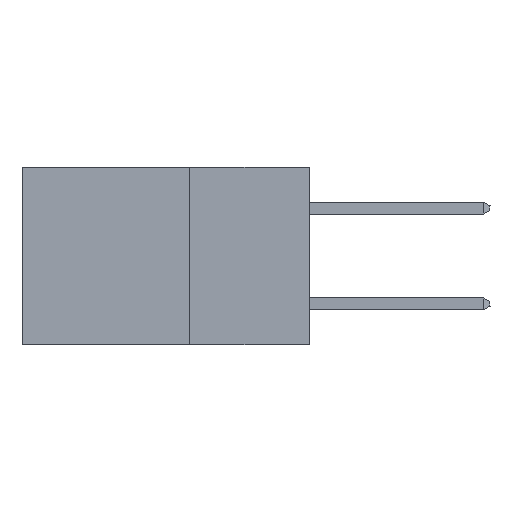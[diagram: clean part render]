
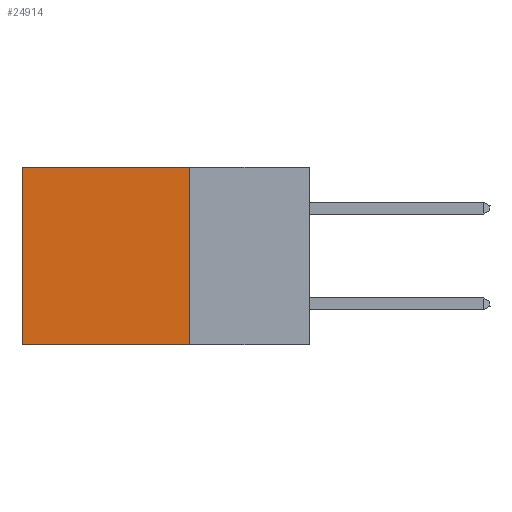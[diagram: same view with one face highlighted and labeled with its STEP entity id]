
A CAD part, left-side view. The second image highlights one B-rep face of the part: STEP entity #24914.
In plain terms, the highlighted planar face has unit normal (-1, 0, 0).
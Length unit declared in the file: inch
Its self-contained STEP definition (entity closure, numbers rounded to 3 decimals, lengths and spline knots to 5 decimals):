
#1022 = VECTOR ( 'NONE', #8077, 39.37008 ) ;
#1148 = EDGE_LOOP ( 'NONE', ( #30023, #14138, #10539, #38861 ) ) ;
#2577 = CARTESIAN_POINT ( 'NONE',  ( 0.2875, 0.25, 0. ) ) ;
#3048 = DIRECTION ( 'NONE',  ( 1., 0., 0. ) ) ;
#4821 = CARTESIAN_POINT ( 'NONE',  ( 0.2875, 0.6, -0.37 ) ) ;
#4990 = CARTESIAN_POINT ( 'NONE',  ( 0.2875, 0.6, 0. ) ) ;
#6301 = VERTEX_POINT ( 'NONE', #31669 ) ;
#6330 = EDGE_CURVE ( 'NONE', #6301, #18238, #8256, .T. ) ;
#6855 = VERTEX_POINT ( 'NONE', #31880 ) ;
#8077 = DIRECTION ( 'NONE',  ( 0., 0., -1. ) ) ;
#8256 = LINE ( 'NONE', #19258, #41388 ) ;
#8545 = DIRECTION ( 'NONE',  ( 0., 1., 0. ) ) ;
#9550 = EDGE_CURVE ( 'NONE', #39861, #6855, #35177, .T. ) ;
#10539 = ORIENTED_EDGE ( 'NONE', *, *, #35698, .F. ) ;
#11587 = CARTESIAN_POINT ( 'NONE',  ( 0.2875, 0.25, 0. ) ) ;
#14138 = ORIENTED_EDGE ( 'NONE', *, *, #6330, .F. ) ;
#17449 = VECTOR ( 'NONE', #8545, 39.37008 ) ;
#18238 = VERTEX_POINT ( 'NONE', #4821 ) ;
#19258 = CARTESIAN_POINT ( 'NONE',  ( 0.2875, 0.25, -0.37 ) ) ;
#19964 = AXIS2_PLACEMENT_3D ( 'NONE', #2577, #3048, #35775 ) ;
#24914 = ADVANCED_FACE ( 'NONE', ( #38401 ), #39150, .F. ) ;
#26422 = CARTESIAN_POINT ( 'NONE',  ( 0.2875, 0.25, 0. ) ) ;
#26456 = EDGE_CURVE ( 'NONE', #6855, #18238, #30261, .T. ) ;
#30023 = ORIENTED_EDGE ( 'NONE', *, *, #26456, .T. ) ;
#30261 = LINE ( 'NONE', #4990, #46245 ) ;
#30712 = LINE ( 'NONE', #26422, #1022 ) ;
#31669 = CARTESIAN_POINT ( 'NONE',  ( 0.2875, 0.25, -0.37 ) ) ;
#31880 = CARTESIAN_POINT ( 'NONE',  ( 0.2875, 0.6, 0. ) ) ;
#34214 = DIRECTION ( 'NONE',  ( 0., 0., -1. ) ) ;
#35177 = LINE ( 'NONE', #11587, #17449 ) ;
#35698 = EDGE_CURVE ( 'NONE', #39861, #6301, #30712, .T. ) ;
#35775 = DIRECTION ( 'NONE',  ( 0., 0., -1. ) ) ;
#37286 = CARTESIAN_POINT ( 'NONE',  ( 0.2875, 0.25, 0. ) ) ;
#38401 = FACE_OUTER_BOUND ( 'NONE', #1148, .T. ) ;
#38861 = ORIENTED_EDGE ( 'NONE', *, *, #9550, .T. ) ;
#39150 = PLANE ( 'NONE',  #19964 ) ;
#39861 = VERTEX_POINT ( 'NONE', #37286 ) ;
#40708 = DIRECTION ( 'NONE',  ( 0., 1., 0. ) ) ;
#41388 = VECTOR ( 'NONE', #40708, 39.37008 ) ;
#46245 = VECTOR ( 'NONE', #34214, 39.37008 ) ;
